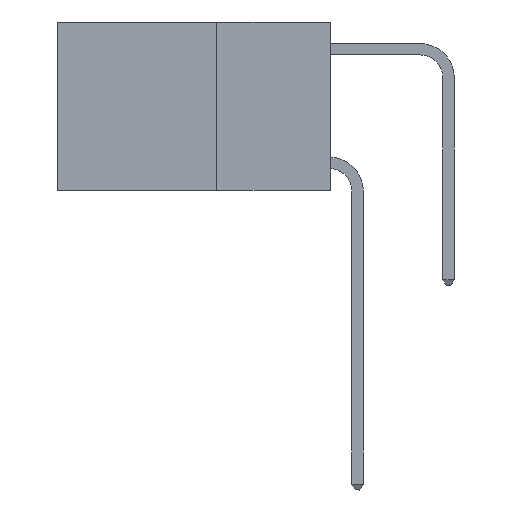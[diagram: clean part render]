
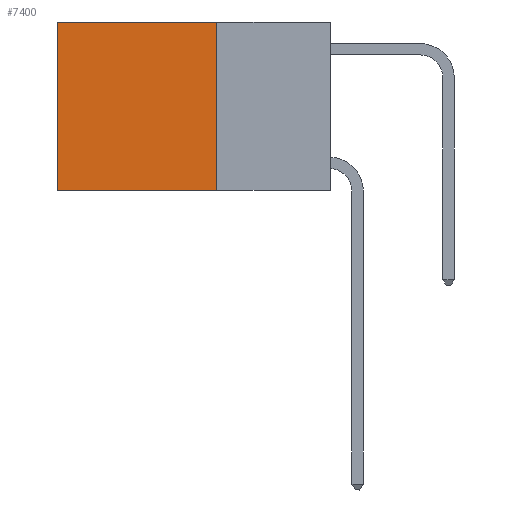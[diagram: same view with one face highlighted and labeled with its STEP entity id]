
A CAD part, left-side view. The second image highlights one B-rep face of the part: STEP entity #7400.
In plain terms, the highlighted planar face has unit normal (-1, 0, 0).
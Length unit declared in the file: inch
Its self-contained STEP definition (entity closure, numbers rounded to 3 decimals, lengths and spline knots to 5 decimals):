
#362 = DIRECTION ( 'NONE',  ( 0., 1., 0. ) ) ;
#712 = EDGE_CURVE ( 'NONE', #13141, #12323, #9254, .T. ) ;
#1560 = CARTESIAN_POINT ( 'NONE',  ( 0.2625, 0.25, 0. ) ) ;
#1643 = VECTOR ( 'NONE', #2209, 39.37008 ) ;
#2209 = DIRECTION ( 'NONE',  ( 0., 1., 0. ) ) ;
#2610 = ORIENTED_EDGE ( 'NONE', *, *, #7113, .F. ) ;
#2632 = DIRECTION ( 'NONE',  ( 0., 0., -1. ) ) ;
#2678 = DIRECTION ( 'NONE',  ( 1., 0., 0. ) ) ;
#2973 = LINE ( 'NONE', #9097, #8708 ) ;
#4135 = VECTOR ( 'NONE', #362, 39.37008 ) ;
#4231 = ORIENTED_EDGE ( 'NONE', *, *, #4459, .T. ) ;
#4459 = EDGE_CURVE ( 'NONE', #12053, #13141, #12378, .T. ) ;
#4552 = LINE ( 'NONE', #7581, #1643 ) ;
#4671 = CARTESIAN_POINT ( 'NONE',  ( 0.2625, 0.6, 0. ) ) ;
#5706 = ORIENTED_EDGE ( 'NONE', *, *, #712, .T. ) ;
#5790 = ORIENTED_EDGE ( 'NONE', *, *, #9639, .F. ) ;
#6017 = VECTOR ( 'NONE', #11913, 39.37008 ) ;
#6196 = EDGE_LOOP ( 'NONE', ( #5706, #2610, #5790, #4231 ) ) ;
#6502 = CARTESIAN_POINT ( 'NONE',  ( 0.2625, 0.6, 0. ) ) ;
#6833 = VERTEX_POINT ( 'NONE', #9316 ) ;
#6877 = CARTESIAN_POINT ( 'NONE',  ( 0.2625, 0.25, 0. ) ) ;
#7113 = EDGE_CURVE ( 'NONE', #6833, #12323, #4552, .T. ) ;
#7400 = ADVANCED_FACE ( 'NONE', ( #12317 ), #8049, .F. ) ;
#7581 = CARTESIAN_POINT ( 'NONE',  ( 0.2625, 0.25, -0.37 ) ) ;
#8049 = PLANE ( 'NONE',  #9307 ) ;
#8674 = CARTESIAN_POINT ( 'NONE',  ( 0.2625, 0.6, -0.37 ) ) ;
#8708 = VECTOR ( 'NONE', #2632, 39.37008 ) ;
#9097 = CARTESIAN_POINT ( 'NONE',  ( 0.2625, 0.25, 0. ) ) ;
#9254 = LINE ( 'NONE', #6502, #6017 ) ;
#9307 = AXIS2_PLACEMENT_3D ( 'NONE', #1560, #2678, #10266 ) ;
#9316 = CARTESIAN_POINT ( 'NONE',  ( 0.2625, 0.25, -0.37 ) ) ;
#9639 = EDGE_CURVE ( 'NONE', #12053, #6833, #2973, .T. ) ;
#10266 = DIRECTION ( 'NONE',  ( 0., 0., -1. ) ) ;
#11518 = CARTESIAN_POINT ( 'NONE',  ( 0.2625, 0.25, 0. ) ) ;
#11913 = DIRECTION ( 'NONE',  ( 0., 0., -1. ) ) ;
#12053 = VERTEX_POINT ( 'NONE', #11518 ) ;
#12317 = FACE_OUTER_BOUND ( 'NONE', #6196, .T. ) ;
#12323 = VERTEX_POINT ( 'NONE', #8674 ) ;
#12378 = LINE ( 'NONE', #6877, #4135 ) ;
#13141 = VERTEX_POINT ( 'NONE', #4671 ) ;
